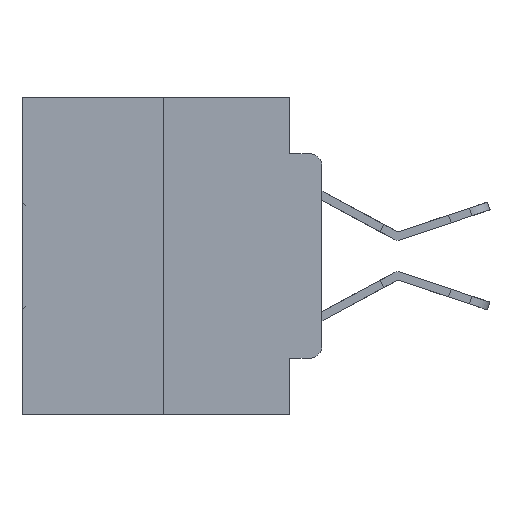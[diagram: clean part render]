
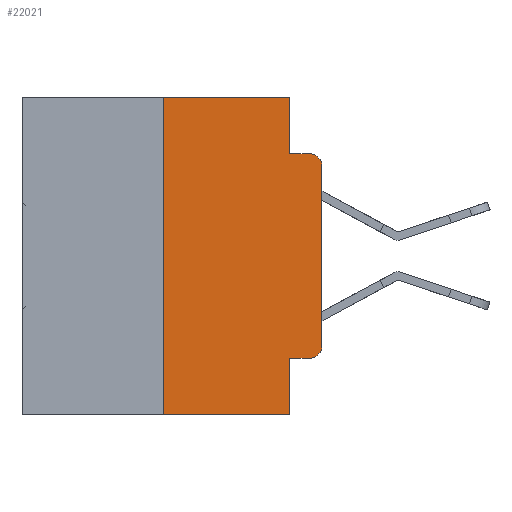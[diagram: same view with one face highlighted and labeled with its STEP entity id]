
A CAD part, left-side view. The second image highlights one B-rep face of the part: STEP entity #22021.
In plain terms, the highlighted planar face has unit normal (-1, 0, 0).
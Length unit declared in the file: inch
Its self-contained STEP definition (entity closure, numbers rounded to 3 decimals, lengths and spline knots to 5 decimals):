
#776 = VERTEX_POINT ( 'NONE', #7048 ) ;
#898 = EDGE_LOOP ( 'NONE', ( #9043, #11796, #32045, #5864, #28668, #25600, #9921, #31472, #26962, #24214 ) ) ;
#1663 = AXIS2_PLACEMENT_3D ( 'NONE', #33317, #9971, #20371 ) ;
#2318 = LINE ( 'NONE', #25202, #7475 ) ;
#2764 = EDGE_CURVE ( 'NONE', #32350, #19301, #13327, .T. ) ;
#3141 = VECTOR ( 'NONE', #18592, 39.37008 ) ;
#3370 = AXIS2_PLACEMENT_3D ( 'NONE', #25608, #30394, #27839 ) ;
#4329 = EDGE_CURVE ( 'NONE', #776, #16406, #6661, .T. ) ;
#5610 = VECTOR ( 'NONE', #33404, 39.37008 ) ;
#5641 = DIRECTION ( 'NONE',  ( 0., 0., -1. ) ) ;
#5864 = ORIENTED_EDGE ( 'NONE', *, *, #31256, .F. ) ;
#6661 = CIRCLE ( 'NONE', #3370, 0.02 ) ;
#7048 = CARTESIAN_POINT ( 'NONE',  ( 0., 0.02, -0.4115 ) ) ;
#7475 = VECTOR ( 'NONE', #10369, 39.37008 ) ;
#7832 = EDGE_CURVE ( 'NONE', #25798, #776, #27598, .T. ) ;
#8721 = DIRECTION ( 'NONE',  ( 0., -1., 0. ) ) ;
#9011 = CARTESIAN_POINT ( 'NONE',  ( 0., 0., -0.1085 ) ) ;
#9043 = ORIENTED_EDGE ( 'NONE', *, *, #20311, .T. ) ;
#9691 = CARTESIAN_POINT ( 'NONE',  ( 0., 0.051, -0.4115 ) ) ;
#9921 = ORIENTED_EDGE ( 'NONE', *, *, #33518, .T. ) ;
#9958 = CARTESIAN_POINT ( 'NONE',  ( 0., 0.051, -0.0885 ) ) ;
#9971 = DIRECTION ( 'NONE',  ( -1., 0., 0. ) ) ;
#10369 = DIRECTION ( 'NONE',  ( 0., 0., -1. ) ) ;
#10988 = DIRECTION ( 'NONE',  ( 0., 0., 1. ) ) ;
#10995 = EDGE_CURVE ( 'NONE', #28039, #31874, #16912, .T. ) ;
#11154 = CARTESIAN_POINT ( 'NONE',  ( 0., 0.473, -0.5 ) ) ;
#11796 = ORIENTED_EDGE ( 'NONE', *, *, #18066, .T. ) ;
#12117 = LINE ( 'NONE', #22997, #5610 ) ;
#12607 = CIRCLE ( 'NONE', #1663, 0.02 ) ;
#12705 = VECTOR ( 'NONE', #10988, 39.37008 ) ;
#13327 = LINE ( 'NONE', #27097, #3141 ) ;
#13883 = DIRECTION ( 'NONE',  ( 0., -1., 0. ) ) ;
#14335 = EDGE_CURVE ( 'NONE', #25798, #17529, #2318, .T. ) ;
#15733 = DIRECTION ( 'NONE',  ( 1., 0., 0. ) ) ;
#16406 = VERTEX_POINT ( 'NONE', #23775 ) ;
#16513 = AXIS2_PLACEMENT_3D ( 'NONE', #20336, #15733, #18448 ) ;
#16912 = LINE ( 'NONE', #30187, #31261 ) ;
#17512 = CARTESIAN_POINT ( 'NONE',  ( 0., 0.25, 0. ) ) ;
#17529 = VERTEX_POINT ( 'NONE', #33186 ) ;
#18066 = EDGE_CURVE ( 'NONE', #22201, #31874, #12607, .T. ) ;
#18443 = VECTOR ( 'NONE', #13883, 39.37008 ) ;
#18448 = DIRECTION ( 'NONE',  ( 0., 0., -1. ) ) ;
#18592 = DIRECTION ( 'NONE',  ( 0., -1., 0. ) ) ;
#19196 = VECTOR ( 'NONE', #30487, 39.37008 ) ;
#19301 = VERTEX_POINT ( 'NONE', #25309 ) ;
#19658 = LINE ( 'NONE', #11154, #18443 ) ;
#20311 = EDGE_CURVE ( 'NONE', #16406, #22201, #12117, .T. ) ;
#20336 = CARTESIAN_POINT ( 'NONE',  ( 0., 0.473, 0. ) ) ;
#20371 = DIRECTION ( 'NONE',  ( 0., 0., -1. ) ) ;
#21716 = CARTESIAN_POINT ( 'NONE',  ( 0., 0.25, 0. ) ) ;
#21782 = EDGE_CURVE ( 'NONE', #32081, #32350, #29380, .T. ) ;
#22021 = ADVANCED_FACE ( 'NONE', ( #25610 ), #25443, .F. ) ;
#22201 = VERTEX_POINT ( 'NONE', #9011 ) ;
#22997 = CARTESIAN_POINT ( 'NONE',  ( 0., 0., 0. ) ) ;
#23775 = CARTESIAN_POINT ( 'NONE',  ( 0., 0., -0.3915 ) ) ;
#24214 = ORIENTED_EDGE ( 'NONE', *, *, #4329, .T. ) ;
#25202 = CARTESIAN_POINT ( 'NONE',  ( 0., 0.051, 0. ) ) ;
#25309 = CARTESIAN_POINT ( 'NONE',  ( 0., 0.051, 0. ) ) ;
#25443 = PLANE ( 'NONE',  #16513 ) ;
#25600 = ORIENTED_EDGE ( 'NONE', *, *, #21782, .F. ) ;
#25608 = CARTESIAN_POINT ( 'NONE',  ( 0., 0.02, -0.3915 ) ) ;
#25610 = FACE_OUTER_BOUND ( 'NONE', #898, .T. ) ;
#25798 = VERTEX_POINT ( 'NONE', #9691 ) ;
#26205 = CARTESIAN_POINT ( 'NONE',  ( 0., 0.25, -0.5 ) ) ;
#26441 = CARTESIAN_POINT ( 'NONE',  ( 0., 0.051, 0. ) ) ;
#26962 = ORIENTED_EDGE ( 'NONE', *, *, #7832, .T. ) ;
#27097 = CARTESIAN_POINT ( 'NONE',  ( 0., 0.473, 0. ) ) ;
#27426 = CARTESIAN_POINT ( 'NONE',  ( 0., 0.02, -0.0885 ) ) ;
#27566 = VECTOR ( 'NONE', #5641, 39.37008 ) ;
#27598 = LINE ( 'NONE', #27773, #19196 ) ;
#27773 = CARTESIAN_POINT ( 'NONE',  ( 0., 0.051, -0.4115 ) ) ;
#27839 = DIRECTION ( 'NONE',  ( 0., 0., -1. ) ) ;
#28039 = VERTEX_POINT ( 'NONE', #9958 ) ;
#28668 = ORIENTED_EDGE ( 'NONE', *, *, #2764, .F. ) ;
#29020 = LINE ( 'NONE', #26441, #27566 ) ;
#29380 = LINE ( 'NONE', #21716, #12705 ) ;
#30187 = CARTESIAN_POINT ( 'NONE',  ( 0., 0.051, -0.0885 ) ) ;
#30394 = DIRECTION ( 'NONE',  ( -1., 0., 0. ) ) ;
#30487 = DIRECTION ( 'NONE',  ( 0., -1., 0. ) ) ;
#31256 = EDGE_CURVE ( 'NONE', #19301, #28039, #29020, .T. ) ;
#31261 = VECTOR ( 'NONE', #8721, 39.37008 ) ;
#31472 = ORIENTED_EDGE ( 'NONE', *, *, #14335, .F. ) ;
#31874 = VERTEX_POINT ( 'NONE', #27426 ) ;
#32045 = ORIENTED_EDGE ( 'NONE', *, *, #10995, .F. ) ;
#32081 = VERTEX_POINT ( 'NONE', #26205 ) ;
#32350 = VERTEX_POINT ( 'NONE', #17512 ) ;
#33186 = CARTESIAN_POINT ( 'NONE',  ( 0., 0.051, -0.5 ) ) ;
#33317 = CARTESIAN_POINT ( 'NONE',  ( 0., 0.02, -0.1085 ) ) ;
#33404 = DIRECTION ( 'NONE',  ( 0., 0., 1. ) ) ;
#33518 = EDGE_CURVE ( 'NONE', #32081, #17529, #19658, .T. ) ;
